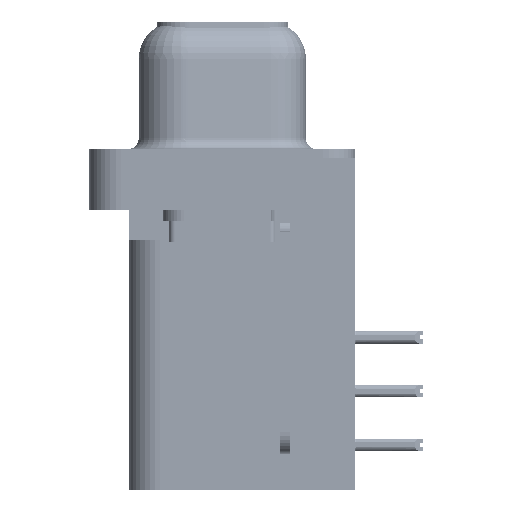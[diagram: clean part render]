
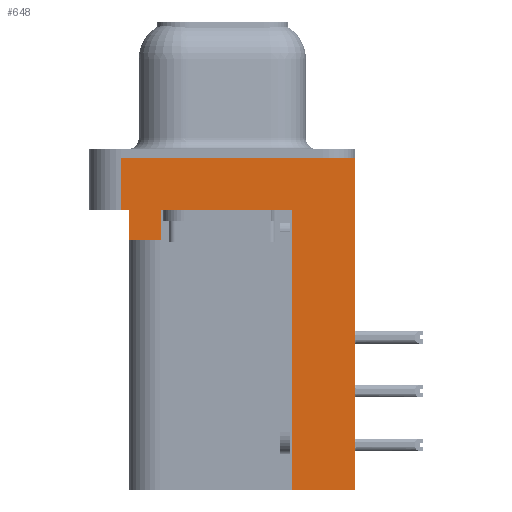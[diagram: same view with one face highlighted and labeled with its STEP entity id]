
A CAD part, left-side view. The second image highlights one B-rep face of the part: STEP entity #648.
In plain terms, the highlighted planar face has unit normal (-1, 0, 0).
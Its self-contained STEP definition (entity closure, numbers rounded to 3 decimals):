
#151 = VERTEX_POINT ( 'NONE', #38256 ) ;
#163 = ORIENTED_EDGE ( 'NONE', *, *, #30755, .T. ) ;
#648 = ADVANCED_FACE ( 'NONE', ( #2667 ), #36579, .T. ) ;
#846 = LINE ( 'NONE', #14428, #35329 ) ;
#1149 = ORIENTED_EDGE ( 'NONE', *, *, #23615, .F. ) ;
#2015 = CARTESIAN_POINT ( 'NONE',  ( -3., 4.425, -3.9 ) ) ;
#2061 = LINE ( 'NONE', #2015, #19239 ) ;
#2667 = FACE_OUTER_BOUND ( 'NONE', #39080, .T. ) ;
#2897 = CARTESIAN_POINT ( 'NONE',  ( -3., -3.295, -15.7 ) ) ;
#2968 = CARTESIAN_POINT ( 'NONE',  ( -3., 2.895, -3.9 ) ) ;
#3156 = ORIENTED_EDGE ( 'NONE', *, *, #23887, .F. ) ;
#3383 = ORIENTED_EDGE ( 'NONE', *, *, #23945, .T. ) ;
#3572 = CARTESIAN_POINT ( 'NONE',  ( -3., -6.275, 0. ) ) ;
#4384 = LINE ( 'NONE', #20000, #21622 ) ;
#5106 = CARTESIAN_POINT ( 'NONE',  ( -3., -3.295, -2.5 ) ) ;
#7421 = VECTOR ( 'NONE', #41091, 1000. ) ;
#8349 = CARTESIAN_POINT ( 'NONE',  ( -3., -3.295, -15.7 ) ) ;
#8352 = VERTEX_POINT ( 'NONE', #23291 ) ;
#8527 = LINE ( 'NONE', #14649, #25764 ) ;
#8557 = ORIENTED_EDGE ( 'NONE', *, *, #32761, .T. ) ;
#9115 = CARTESIAN_POINT ( 'NONE',  ( -3., 4.425, -3.9 ) ) ;
#9473 = DIRECTION ( 'NONE',  ( 0., 0., 1. ) ) ;
#12251 = CARTESIAN_POINT ( 'NONE',  ( -3., -6.275, -2.5 ) ) ;
#12591 = DIRECTION ( 'NONE',  ( 0., 1., 0. ) ) ;
#13351 = DIRECTION ( 'NONE',  ( 0., 0., 1. ) ) ;
#13718 = DIRECTION ( 'NONE',  ( 0., 0., 1. ) ) ;
#14408 = LINE ( 'NONE', #37863, #32727 ) ;
#14428 = CARTESIAN_POINT ( 'NONE',  ( -3., -6.275, -2.5 ) ) ;
#14649 = CARTESIAN_POINT ( 'NONE',  ( -3., 4.775, -2.5 ) ) ;
#15009 = AXIS2_PLACEMENT_3D ( 'NONE', #12251, #19501, #9473 ) ;
#16544 = LINE ( 'NONE', #40934, #7421 ) ;
#17393 = DIRECTION ( 'NONE',  ( 0., -1., 0. ) ) ;
#17448 = VERTEX_POINT ( 'NONE', #5106 ) ;
#17816 = VECTOR ( 'NONE', #12591, 1000. ) ;
#18110 = VERTEX_POINT ( 'NONE', #19625 ) ;
#18219 = VERTEX_POINT ( 'NONE', #44476 ) ;
#19239 = VECTOR ( 'NONE', #39949, 1000. ) ;
#19501 = DIRECTION ( 'NONE',  ( -1., 0., 0. ) ) ;
#19625 = CARTESIAN_POINT ( 'NONE',  ( -3., 2.895, -2.5 ) ) ;
#20000 = CARTESIAN_POINT ( 'NONE',  ( -3., -6.275, -2.5 ) ) ;
#20559 = DIRECTION ( 'NONE',  ( 0., 0., 1. ) ) ;
#20856 = ORIENTED_EDGE ( 'NONE', *, *, #34101, .T. ) ;
#21103 = VERTEX_POINT ( 'NONE', #21166 ) ;
#21166 = CARTESIAN_POINT ( 'NONE',  ( -3., 2.895, -3.9 ) ) ;
#21388 = VERTEX_POINT ( 'NONE', #21927 ) ;
#21460 = VECTOR ( 'NONE', #17393, 1000. ) ;
#21622 = VECTOR ( 'NONE', #44404, 1000. ) ;
#21927 = CARTESIAN_POINT ( 'NONE',  ( -3., 4.425, -3.9 ) ) ;
#22402 = VECTOR ( 'NONE', #13351, 1000. ) ;
#22839 = ORIENTED_EDGE ( 'NONE', *, *, #26546, .F. ) ;
#23291 = CARTESIAN_POINT ( 'NONE',  ( -3., 4.425, -2.5 ) ) ;
#23342 = EDGE_CURVE ( 'NONE', #27786, #18219, #8527, .T. ) ;
#23549 = EDGE_CURVE ( 'NONE', #21388, #8352, #2061, .T. ) ;
#23615 = EDGE_CURVE ( 'NONE', #28254, #17448, #26268, .T. ) ;
#23887 = EDGE_CURVE ( 'NONE', #151, #28254, #16544, .T. ) ;
#23945 = EDGE_CURVE ( 'NONE', #151, #29208, #14408, .T. ) ;
#25764 = VECTOR ( 'NONE', #35349, 1000. ) ;
#26268 = LINE ( 'NONE', #2897, #37722 ) ;
#26546 = EDGE_CURVE ( 'NONE', #18219, #29208, #41031, .T. ) ;
#27786 = VERTEX_POINT ( 'NONE', #39702 ) ;
#28167 = DIRECTION ( 'NONE',  ( 0., -1., 0. ) ) ;
#28254 = VERTEX_POINT ( 'NONE', #8349 ) ;
#29208 = VERTEX_POINT ( 'NONE', #42520 ) ;
#30755 = EDGE_CURVE ( 'NONE', #27786, #8352, #4384, .T. ) ;
#31164 = EDGE_CURVE ( 'NONE', #21103, #21388, #44513, .T. ) ;
#31581 = LINE ( 'NONE', #2968, #22402 ) ;
#32727 = VECTOR ( 'NONE', #20559, 1000. ) ;
#32761 = EDGE_CURVE ( 'NONE', #21103, #18110, #31581, .T. ) ;
#34101 = EDGE_CURVE ( 'NONE', #18110, #17448, #846, .T. ) ;
#35329 = VECTOR ( 'NONE', #28167, 1000. ) ;
#35349 = DIRECTION ( 'NONE',  ( 0., 0., 1. ) ) ;
#36579 = PLANE ( 'NONE',  #15009 ) ;
#36594 = ORIENTED_EDGE ( 'NONE', *, *, #31164, .F. ) ;
#37722 = VECTOR ( 'NONE', #13718, 1000. ) ;
#37863 = CARTESIAN_POINT ( 'NONE',  ( -3., -6.275, -2.5 ) ) ;
#38256 = CARTESIAN_POINT ( 'NONE',  ( -3., -6.275, -15.7 ) ) ;
#39080 = EDGE_LOOP ( 'NONE', ( #22839, #39719, #163, #43033, #36594, #8557, #20856, #1149, #3156, #3383 ) ) ;
#39702 = CARTESIAN_POINT ( 'NONE',  ( -3., 4.775, -2.5 ) ) ;
#39719 = ORIENTED_EDGE ( 'NONE', *, *, #23342, .F. ) ;
#39949 = DIRECTION ( 'NONE',  ( 0., 0., 1. ) ) ;
#40934 = CARTESIAN_POINT ( 'NONE',  ( -3., -3.295, -15.7 ) ) ;
#41031 = LINE ( 'NONE', #3572, #21460 ) ;
#41091 = DIRECTION ( 'NONE',  ( 0., 1., 0. ) ) ;
#42520 = CARTESIAN_POINT ( 'NONE',  ( -3., -6.275, 0. ) ) ;
#43033 = ORIENTED_EDGE ( 'NONE', *, *, #23549, .F. ) ;
#44404 = DIRECTION ( 'NONE',  ( 0., -1., 0. ) ) ;
#44476 = CARTESIAN_POINT ( 'NONE',  ( -3., 4.775, 0. ) ) ;
#44513 = LINE ( 'NONE', #9115, #17816 ) ;
